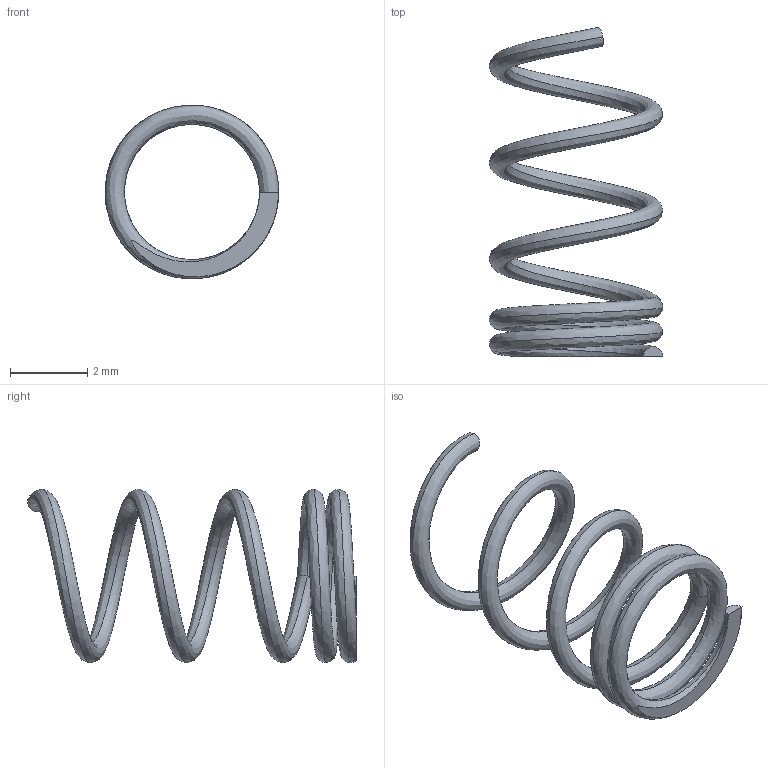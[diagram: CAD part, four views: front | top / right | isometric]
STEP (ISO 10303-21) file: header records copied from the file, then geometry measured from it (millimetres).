
FILE_DESCRIPTION (( 'STEP AP214' ), '1' );
FILE_NAME ('Barrel_Lock_Spring.step', '2013-11-06T14:30:51', ( 'elpi' ), ( '' ), 'SwSTEP 2.0', 'SolidWorks 2013', '' );
FILE_SCHEMA (( 'AUTOMOTIVE_DESIGN' ));
Length unit declared in the file: millimetre
Products named in the file (1): Barrel_Lock_Spring
Bounding box: 4.5 x 8.52 x 4.5 mm (x, y, z)
Volume: 11.8 mm3; surface area: 95.8 mm2
Topology: 1 solids, 1 shells, 7 faces, 11 edges, 6 vertices
Faces by surface type: bspline 4, plane 3
Entity records: 2635 total; most frequent: CARTESIAN_POINT 2510, ORIENTED_EDGE 22, DIRECTION 11, EDGE_CURVE 11, FACE_OUTER_BOUND 7, ADVANCED_FACE 7, EDGE_LOOP 7, VERTEX_POINT 6
